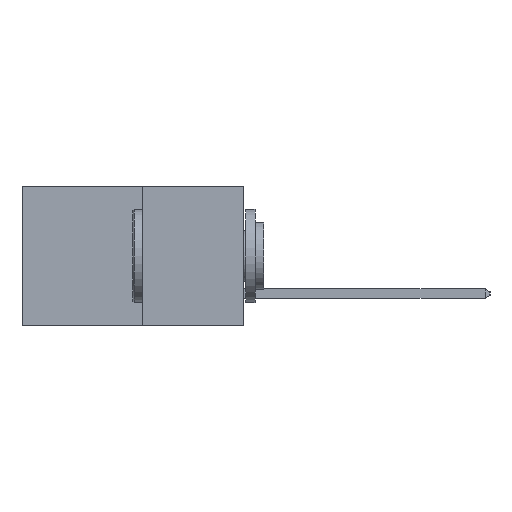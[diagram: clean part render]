
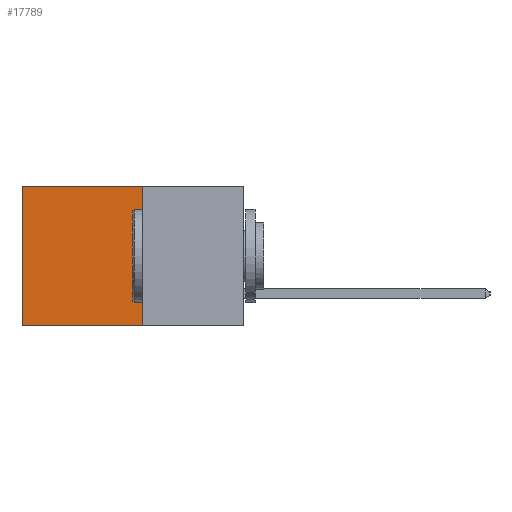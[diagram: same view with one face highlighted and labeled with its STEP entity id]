
A CAD part, left-side view. The second image highlights one B-rep face of the part: STEP entity #17789.
In plain terms, the highlighted planar face has unit normal (-1, 0, 0).
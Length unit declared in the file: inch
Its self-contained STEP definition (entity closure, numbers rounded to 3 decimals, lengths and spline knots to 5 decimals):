
#77 = VERTEX_POINT ( 'NONE', #26156 ) ;
#1923 = VERTEX_POINT ( 'NONE', #11765 ) ;
#3074 = ORIENTED_EDGE ( 'NONE', *, *, #7240, .T. ) ;
#3477 = VECTOR ( 'NONE', #23913, 39.37008 ) ;
#3489 = ORIENTED_EDGE ( 'NONE', *, *, #4401, .F. ) ;
#4157 = LINE ( 'NONE', #24016, #3477 ) ;
#4401 = EDGE_CURVE ( 'NONE', #1923, #77, #16486, .T. ) ;
#4905 = EDGE_CURVE ( 'NONE', #20661, #77, #4157, .T. ) ;
#5477 = VECTOR ( 'NONE', #8607, 39.37008 ) ;
#6418 = CARTESIAN_POINT ( 'NONE',  ( 0.277, 0.27, -0.37 ) ) ;
#7240 = EDGE_CURVE ( 'NONE', #26801, #20661, #14268, .T. ) ;
#8607 = DIRECTION ( 'NONE',  ( 0., 0., -1. ) ) ;
#9324 = DIRECTION ( 'NONE',  ( 1., 0., 0. ) ) ;
#9934 = FACE_OUTER_BOUND ( 'NONE', #27641, .T. ) ;
#11189 = EDGE_CURVE ( 'NONE', #26801, #1923, #17743, .T. ) ;
#11765 = CARTESIAN_POINT ( 'NONE',  ( 0.277, 0.27, -0.37 ) ) ;
#12213 = DIRECTION ( 'NONE',  ( 0., 1., 0. ) ) ;
#14063 = CARTESIAN_POINT ( 'NONE',  ( 0.277, 0.27, -0.37 ) ) ;
#14065 = DIRECTION ( 'NONE',  ( 0., 1., 0. ) ) ;
#14268 = LINE ( 'NONE', #27191, #25054 ) ;
#16486 = LINE ( 'NONE', #14063, #22873 ) ;
#17743 = LINE ( 'NONE', #6418, #5477 ) ;
#17789 = ADVANCED_FACE ( 'NONE', ( #9934 ), #26514, .F. ) ;
#17908 = ORIENTED_EDGE ( 'NONE', *, *, #4905, .T. ) ;
#18498 = CARTESIAN_POINT ( 'NONE',  ( 0.277, 0.59, 0. ) ) ;
#19832 = CARTESIAN_POINT ( 'NONE',  ( 0.277, 0.27, 0. ) ) ;
#20661 = VERTEX_POINT ( 'NONE', #18498 ) ;
#22000 = ORIENTED_EDGE ( 'NONE', *, *, #11189, .F. ) ;
#22286 = CARTESIAN_POINT ( 'NONE',  ( 0.277, 0.27, -0.37 ) ) ;
#22873 = VECTOR ( 'NONE', #14065, 39.37008 ) ;
#23913 = DIRECTION ( 'NONE',  ( 0., 0., -1. ) ) ;
#24016 = CARTESIAN_POINT ( 'NONE',  ( 0.277, 0.59, -0.37 ) ) ;
#24465 = DIRECTION ( 'NONE',  ( 0., 0., -1. ) ) ;
#25054 = VECTOR ( 'NONE', #12213, 39.37008 ) ;
#26156 = CARTESIAN_POINT ( 'NONE',  ( 0.277, 0.59, -0.37 ) ) ;
#26438 = AXIS2_PLACEMENT_3D ( 'NONE', #22286, #9324, #24465 ) ;
#26514 = PLANE ( 'NONE',  #26438 ) ;
#26801 = VERTEX_POINT ( 'NONE', #19832 ) ;
#27191 = CARTESIAN_POINT ( 'NONE',  ( 0.277, 0.27, 0. ) ) ;
#27641 = EDGE_LOOP ( 'NONE', ( #17908, #3489, #22000, #3074 ) ) ;
